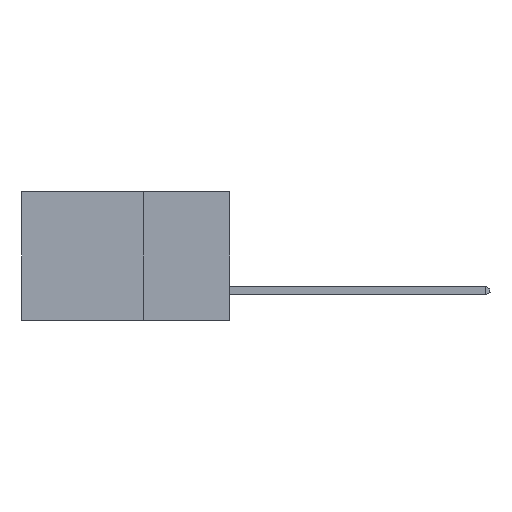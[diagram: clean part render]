
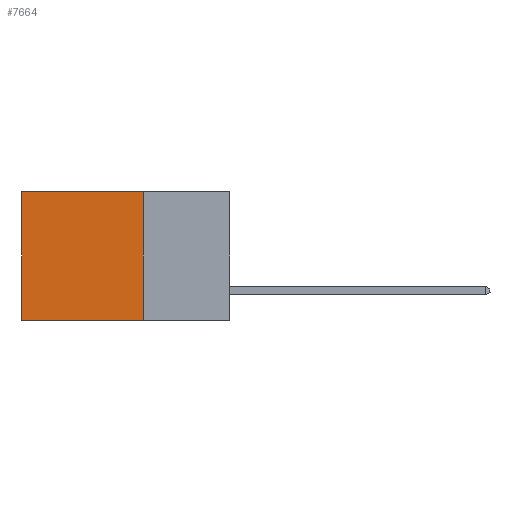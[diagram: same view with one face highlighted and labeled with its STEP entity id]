
A CAD part, left-side view. The second image highlights one B-rep face of the part: STEP entity #7664.
In plain terms, the highlighted planar face has unit normal (-1, 0, 0).
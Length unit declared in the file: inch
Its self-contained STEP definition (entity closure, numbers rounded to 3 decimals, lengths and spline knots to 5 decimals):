
#1094 = FACE_OUTER_BOUND ( 'NONE', #16702, .T. ) ;
#3168 = ORIENTED_EDGE ( 'NONE', *, *, #5636, .T. ) ;
#3401 = DIRECTION ( 'NONE',  ( 0., 0., -1. ) ) ;
#3874 = EDGE_CURVE ( 'NONE', #23557, #16542, #24705, .T. ) ;
#4659 = CARTESIAN_POINT ( 'NONE',  ( 0.298, 0.25, -0.37 ) ) ;
#4826 = VERTEX_POINT ( 'NONE', #9961 ) ;
#5636 = EDGE_CURVE ( 'NONE', #4826, #23557, #15641, .T. ) ;
#6200 = DIRECTION ( 'NONE',  ( 0., 0., -1. ) ) ;
#6331 = AXIS2_PLACEMENT_3D ( 'NONE', #10774, #20005, #6200 ) ;
#6470 = VERTEX_POINT ( 'NONE', #4659 ) ;
#7664 = ADVANCED_FACE ( 'NONE', ( #1094 ), #17726, .F. ) ;
#8033 = VECTOR ( 'NONE', #20934, 39.37008 ) ;
#9217 = LINE ( 'NONE', #24526, #13906 ) ;
#9668 = CARTESIAN_POINT ( 'NONE',  ( 0.298, 0.6, -0.37 ) ) ;
#9961 = CARTESIAN_POINT ( 'NONE',  ( 0.298, 0.25, 0. ) ) ;
#10774 = CARTESIAN_POINT ( 'NONE',  ( 0.298, 0.25, 0. ) ) ;
#12018 = CARTESIAN_POINT ( 'NONE',  ( 0.298, 0.25, 0. ) ) ;
#12598 = EDGE_CURVE ( 'NONE', #4826, #6470, #20419, .T. ) ;
#12613 = VECTOR ( 'NONE', #3401, 39.37008 ) ;
#13602 = VECTOR ( 'NONE', #23164, 39.37008 ) ;
#13906 = VECTOR ( 'NONE', #17843, 39.37008 ) ;
#14301 = EDGE_CURVE ( 'NONE', #6470, #16542, #9217, .T. ) ;
#14732 = ORIENTED_EDGE ( 'NONE', *, *, #12598, .F. ) ;
#15641 = LINE ( 'NONE', #12018, #8033 ) ;
#16317 = CARTESIAN_POINT ( 'NONE',  ( 0.298, 0.25, 0. ) ) ;
#16542 = VERTEX_POINT ( 'NONE', #9668 ) ;
#16702 = EDGE_LOOP ( 'NONE', ( #17011, #25598, #14732, #3168 ) ) ;
#17011 = ORIENTED_EDGE ( 'NONE', *, *, #3874, .T. ) ;
#17726 = PLANE ( 'NONE',  #6331 ) ;
#17843 = DIRECTION ( 'NONE',  ( 0., 1., 0. ) ) ;
#19738 = CARTESIAN_POINT ( 'NONE',  ( 0.298, 0.6, 0. ) ) ;
#20005 = DIRECTION ( 'NONE',  ( 1., 0., 0. ) ) ;
#20419 = LINE ( 'NONE', #16317, #13602 ) ;
#20934 = DIRECTION ( 'NONE',  ( 0., 1., 0. ) ) ;
#21781 = CARTESIAN_POINT ( 'NONE',  ( 0.298, 0.6, 0. ) ) ;
#23164 = DIRECTION ( 'NONE',  ( 0., 0., -1. ) ) ;
#23557 = VERTEX_POINT ( 'NONE', #19738 ) ;
#24526 = CARTESIAN_POINT ( 'NONE',  ( 0.298, 0.25, -0.37 ) ) ;
#24705 = LINE ( 'NONE', #21781, #12613 ) ;
#25598 = ORIENTED_EDGE ( 'NONE', *, *, #14301, .F. ) ;
